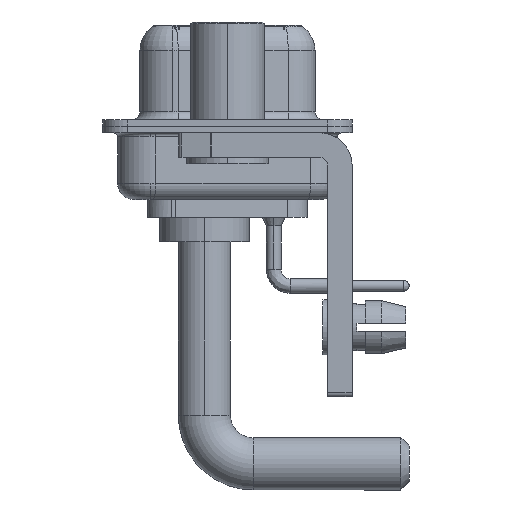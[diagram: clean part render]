
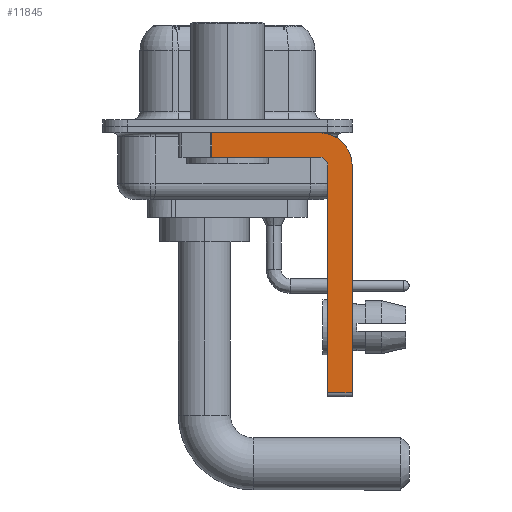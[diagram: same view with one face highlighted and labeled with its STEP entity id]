
A CAD part, left-side view. The second image highlights one B-rep face of the part: STEP entity #11845.
In plain terms, the highlighted planar face has unit normal (-1, 0, 0).
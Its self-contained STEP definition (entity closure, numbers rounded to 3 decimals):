
#292 = EDGE_LOOP ( 'NONE', ( #6308, #8355, #2581, #10963, #2528, #16292, #14369, #19532 ) ) ;
#846 = DIRECTION ( 'NONE',  ( 0., 0., 1. ) ) ;
#925 = DIRECTION ( 'NONE',  ( 0., 0., -1. ) ) ;
#1088 = DIRECTION ( 'NONE',  ( 0., 0., 1. ) ) ;
#1251 = LINE ( 'NONE', #18153, #12322 ) ;
#1537 = DIRECTION ( 'NONE',  ( 0., -1., 0. ) ) ;
#2528 = ORIENTED_EDGE ( 'NONE', *, *, #16166, .F. ) ;
#2581 = ORIENTED_EDGE ( 'NONE', *, *, #17163, .F. ) ;
#2611 = LINE ( 'NONE', #10630, #19137 ) ;
#2659 = CARTESIAN_POINT ( 'NONE',  ( -2.9, 0.978, -1.9 ) ) ;
#2862 = CARTESIAN_POINT ( 'NONE',  ( -2.9, -6.15, -2.4 ) ) ;
#3872 = EDGE_CURVE ( 'NONE', #6767, #12345, #19787, .T. ) ;
#3873 = VERTEX_POINT ( 'NONE', #18243 ) ;
#4442 = VERTEX_POINT ( 'NONE', #18438 ) ;
#4452 = LINE ( 'NONE', #4704, #12942 ) ;
#4704 = CARTESIAN_POINT ( 'NONE',  ( -2.9, -7.65, -2.4 ) ) ;
#5069 = CARTESIAN_POINT ( 'NONE',  ( -2.9, -5.65, -16.35 ) ) ;
#6024 = VERTEX_POINT ( 'NONE', #23804 ) ;
#6308 = ORIENTED_EDGE ( 'NONE', *, *, #8479, .F. ) ;
#6767 = VERTEX_POINT ( 'NONE', #2862 ) ;
#6889 = CIRCLE ( 'NONE', #24097, 2. ) ;
#7282 = DIRECTION ( 'NONE',  ( 1., 0., 0. ) ) ;
#8335 = EDGE_CURVE ( 'NONE', #4442, #3873, #6889, .T. ) ;
#8355 = ORIENTED_EDGE ( 'NONE', *, *, #14102, .T. ) ;
#8479 = EDGE_CURVE ( 'NONE', #15189, #4442, #17417, .T. ) ;
#8732 = CARTESIAN_POINT ( 'NONE',  ( -2.9, -5.65, -2.4 ) ) ;
#9188 = PLANE ( 'NONE',  #19013 ) ;
#10585 = AXIS2_PLACEMENT_3D ( 'NONE', #8732, #14598, #1088 ) ;
#10630 = CARTESIAN_POINT ( 'NONE',  ( -2.9, -6.15, -16.6 ) ) ;
#10717 = VERTEX_POINT ( 'NONE', #14524 ) ;
#10963 = ORIENTED_EDGE ( 'NONE', *, *, #3872, .F. ) ;
#11065 = LINE ( 'NONE', #5069, #21212 ) ;
#11845 = ADVANCED_FACE ( 'NONE', ( #14311 ), #9188, .F. ) ;
#12182 = VERTEX_POINT ( 'NONE', #2659 ) ;
#12322 = VECTOR ( 'NONE', #24168, 1000. ) ;
#12345 = VERTEX_POINT ( 'NONE', #14653 ) ;
#12942 = VECTOR ( 'NONE', #925, 1000. ) ;
#13662 = CARTESIAN_POINT ( 'NONE',  ( -2.9, 3., -0.4 ) ) ;
#14102 = EDGE_CURVE ( 'NONE', #15189, #12182, #1251, .T. ) ;
#14311 = FACE_OUTER_BOUND ( 'NONE', #292, .T. ) ;
#14369 = ORIENTED_EDGE ( 'NONE', *, *, #22161, .F. ) ;
#14524 = CARTESIAN_POINT ( 'NONE',  ( -2.9, -7.65, -16.35 ) ) ;
#14543 = LINE ( 'NONE', #18324, #17571 ) ;
#14598 = DIRECTION ( 'NONE',  ( -1., 0., 0. ) ) ;
#14653 = CARTESIAN_POINT ( 'NONE',  ( -2.9, -5.65, -1.9 ) ) ;
#14670 = VECTOR ( 'NONE', #23559, 1000. ) ;
#14805 = DIRECTION ( 'NONE',  ( 1., 0., 0. ) ) ;
#14917 = DIRECTION ( 'NONE',  ( 0., 0., -1. ) ) ;
#15189 = VERTEX_POINT ( 'NONE', #18918 ) ;
#16166 = EDGE_CURVE ( 'NONE', #6024, #6767, #2611, .T. ) ;
#16176 = DIRECTION ( 'NONE',  ( 0., 1., 0. ) ) ;
#16292 = ORIENTED_EDGE ( 'NONE', *, *, #18114, .T. ) ;
#17163 = EDGE_CURVE ( 'NONE', #12345, #12182, #14543, .T. ) ;
#17417 = LINE ( 'NONE', #13662, #14670 ) ;
#17571 = VECTOR ( 'NONE', #16176, 1000. ) ;
#18114 = EDGE_CURVE ( 'NONE', #6024, #10717, #11065, .T. ) ;
#18153 = CARTESIAN_POINT ( 'NONE',  ( -2.9, 0.978, -1.9 ) ) ;
#18243 = CARTESIAN_POINT ( 'NONE',  ( -2.9, -7.65, -2.4 ) ) ;
#18324 = CARTESIAN_POINT ( 'NONE',  ( -2.9, -5.65, -1.9 ) ) ;
#18438 = CARTESIAN_POINT ( 'NONE',  ( -2.9, -5.65, -0.4 ) ) ;
#18578 = CARTESIAN_POINT ( 'NONE',  ( -2.9, -5.65, -2.4 ) ) ;
#18918 = CARTESIAN_POINT ( 'NONE',  ( -2.9, 0.978, -0.4 ) ) ;
#19013 = AXIS2_PLACEMENT_3D ( 'NONE', #18578, #14805, #24216 ) ;
#19137 = VECTOR ( 'NONE', #846, 1000. ) ;
#19532 = ORIENTED_EDGE ( 'NONE', *, *, #8335, .F. ) ;
#19787 = CIRCLE ( 'NONE', #10585, 0.5 ) ;
#21212 = VECTOR ( 'NONE', #1537, 1000. ) ;
#22161 = EDGE_CURVE ( 'NONE', #3873, #10717, #4452, .T. ) ;
#23559 = DIRECTION ( 'NONE',  ( 0., -1., 0. ) ) ;
#23804 = CARTESIAN_POINT ( 'NONE',  ( -2.9, -6.15, -16.35 ) ) ;
#24097 = AXIS2_PLACEMENT_3D ( 'NONE', #24684, #7282, #14917 ) ;
#24168 = DIRECTION ( 'NONE',  ( 0., 0., -1. ) ) ;
#24216 = DIRECTION ( 'NONE',  ( 0., 0., -1. ) ) ;
#24684 = CARTESIAN_POINT ( 'NONE',  ( -2.9, -5.65, -2.4 ) ) ;
